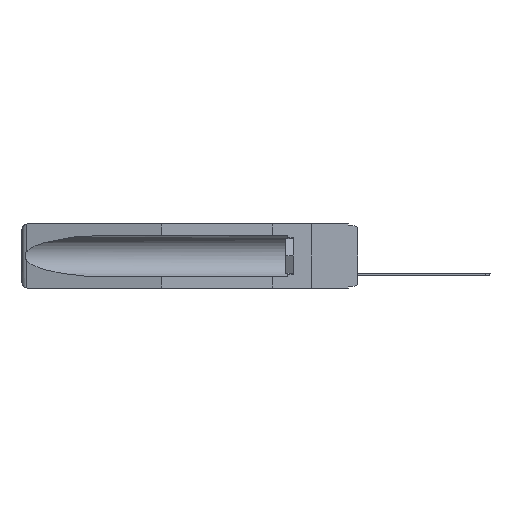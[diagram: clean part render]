
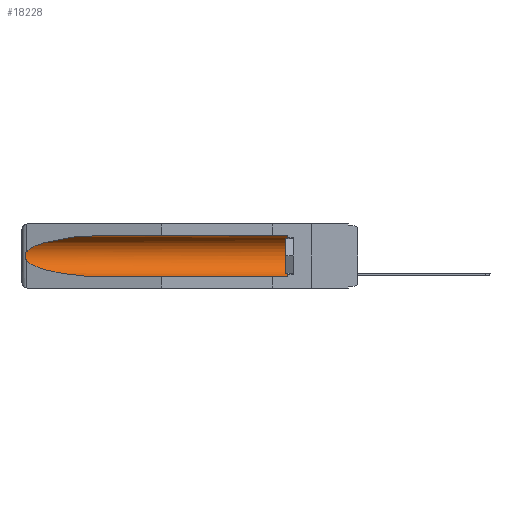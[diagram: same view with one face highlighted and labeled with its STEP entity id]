
A CAD part, left-side view. The second image highlights one B-rep face of the part: STEP entity #18228.
In plain terms, the highlighted cylindrical face has radius 2.857 mm (diameter 5.715 mm), a partial arc.
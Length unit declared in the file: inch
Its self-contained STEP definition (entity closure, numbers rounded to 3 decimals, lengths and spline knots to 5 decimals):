
#122 = CARTESIAN_POINT ( 'NONE',  ( 0.26655, 1.53094, -0.18657 ) ) ;
#272 = ORIENTED_EDGE ( 'NONE', *, *, #1466, .T. ) ;
#1155 =( BOUNDED_CURVE ( )  B_SPLINE_CURVE ( 3, ( #14566, #16086, #17677, #19232 ),
 .UNSPECIFIED., .F., .F. ) 
 B_SPLINE_CURVE_WITH_KNOTS ( ( 4, 4 ),
 ( 0.1948, 1.5708 ),
 .UNSPECIFIED. ) 
 CURVE ( )  GEOMETRIC_REPRESENTATION_ITEM ( )  RATIONAL_B_SPLINE_CURVE ( ( 1., 0.848, 0.848, 1. ) ) 
 REPRESENTATION_ITEM ( '' )  );
#1324 = EDGE_CURVE ( 'NONE', #3491, #7017, #8730, .T. ) ;
#1466 = EDGE_CURVE ( 'NONE', #7017, #9314, #1155, .T. ) ;
#1470 = EDGE_CURVE ( 'NONE', #11580, #15177, #7109, .T. ) ;
#1923 = DIRECTION ( 'NONE',  ( 0., 0., 1. ) ) ;
#1943 = CARTESIAN_POINT ( 'NONE',  ( 0.2673, 1.53269, -0.17917 ) ) ;
#2380 = EDGE_CURVE ( 'NONE', #3036, #3491, #6882, .T. ) ;
#3036 = VERTEX_POINT ( 'NONE', #14897 ) ;
#3089 = EDGE_LOOP ( 'NONE', ( #8557, #5424, #272, #16169, #5481, #16706 ) ) ;
#3181 = AXIS2_PLACEMENT_3D ( 'NONE', #5128, #15964, #6701 ) ;
#3491 = VERTEX_POINT ( 'NONE', #13835 ) ;
#3527 = EDGE_CURVE ( 'NONE', #15177, #3036, #13097, .T. ) ;
#3569 = CARTESIAN_POINT ( 'NONE',  ( 0.155, -0.30754, -0.284 ) ) ;
#4928 = CARTESIAN_POINT ( 'NONE',  ( 0.26537, 1.52718, -0.14972 ) ) ;
#4977 = CARTESIAN_POINT ( 'NONE',  ( 0.155, -0.30754, -0.1715 ) ) ;
#5066 = CARTESIAN_POINT ( 'NONE',  ( 0.26597, 1.5296, -0.19026 ) ) ;
#5128 = CARTESIAN_POINT ( 'NONE',  ( 0.155, 0.126, -0.1715 ) ) ;
#5424 = ORIENTED_EDGE ( 'NONE', *, *, #1324, .T. ) ;
#5481 = ORIENTED_EDGE ( 'NONE', *, *, #1470, .T. ) ;
#5867 = LINE ( 'NONE', #3569, #11201 ) ;
#6054 = VECTOR ( 'NONE', #11794, 39.37008 ) ;
#6504 = CARTESIAN_POINT ( 'NONE',  ( 0.2675, 1.53308, -0.17534 ) ) ;
#6701 = DIRECTION ( 'NONE',  ( 0., 0., 1. ) ) ;
#6882 =( BOUNDED_CURVE ( )  B_SPLINE_CURVE ( 3, ( #18643, #17214, #15638, #9555 ),
 .UNSPECIFIED., .F., .F. ) 
 B_SPLINE_CURVE_WITH_KNOTS ( ( 4, 4 ),
 ( 4.71239, 6.08839 ),
 .UNSPECIFIED. ) 
 CURVE ( )  GEOMETRIC_REPRESENTATION_ITEM ( )  RATIONAL_B_SPLINE_CURVE ( ( 1., 0.848, 0.848, 1. ) ) 
 REPRESENTATION_ITEM ( '' )  );
#7017 = VERTEX_POINT ( 'NONE', #7634 ) ;
#7109 = CIRCLE ( 'NONE', #3181, 0.1125 ) ;
#7634 = CARTESIAN_POINT ( 'NONE',  ( 0.26537, 1.52718, -0.19328 ) ) ;
#8288 = CARTESIAN_POINT ( 'NONE',  ( 0.155, 0.126, -0.059 ) ) ;
#8557 = ORIENTED_EDGE ( 'NONE', *, *, #2380, .T. ) ;
#8730 = B_SPLINE_CURVE_WITH_KNOTS ( 'NONE', 3,
 ( #4928, #9677, #11246, #15752, #12545, #6504, #1943, #122, #5066, #9608 ),
 .UNSPECIFIED., .F., .F.,
 ( 4, 2, 2, 2, 4 ),
 ( 0., 0.00029, 0.00058, 0.00087, 0.00117 ),
 .UNSPECIFIED. ) ;
#9314 = VERTEX_POINT ( 'NONE', #17387 ) ;
#9555 = CARTESIAN_POINT ( 'NONE',  ( 0.26537, 1.52718, -0.14972 ) ) ;
#9608 = CARTESIAN_POINT ( 'NONE',  ( 0.26537, 1.52718, -0.19328 ) ) ;
#9677 = CARTESIAN_POINT ( 'NONE',  ( 0.26597, 1.52961, -0.15275 ) ) ;
#9708 = FACE_OUTER_BOUND ( 'NONE', #3089, .T. ) ;
#9852 = DIRECTION ( 'NONE',  ( 0., 1., 0. ) ) ;
#10766 = AXIS2_PLACEMENT_3D ( 'NONE', #4977, #9852, #1923 ) ;
#10986 = CARTESIAN_POINT ( 'NONE',  ( 0.155, -0.30754, -0.059 ) ) ;
#11201 = VECTOR ( 'NONE', #15965, 39.37008 ) ;
#11246 = CARTESIAN_POINT ( 'NONE',  ( 0.26654, 1.53092, -0.15636 ) ) ;
#11580 = VERTEX_POINT ( 'NONE', #17138 ) ;
#11794 = DIRECTION ( 'NONE',  ( 0., 1., 0. ) ) ;
#12545 = CARTESIAN_POINT ( 'NONE',  ( 0.2675, 1.53308, -0.16763 ) ) ;
#13097 = LINE ( 'NONE', #10986, #6054 ) ;
#13583 = CYLINDRICAL_SURFACE ( 'NONE', #10766, 0.1125 ) ;
#13835 = CARTESIAN_POINT ( 'NONE',  ( 0.26537, 1.52718, -0.14972 ) ) ;
#14566 = CARTESIAN_POINT ( 'NONE',  ( 0.26537, 1.52718, -0.19328 ) ) ;
#14897 = CARTESIAN_POINT ( 'NONE',  ( 0.155, 1.07973, -0.059 ) ) ;
#15177 = VERTEX_POINT ( 'NONE', #8288 ) ;
#15638 = CARTESIAN_POINT ( 'NONE',  ( 0.25451, 1.48313, -0.09465 ) ) ;
#15752 = CARTESIAN_POINT ( 'NONE',  ( 0.2673, 1.5327, -0.16383 ) ) ;
#15964 = DIRECTION ( 'NONE',  ( 0., -1., 0. ) ) ;
#15965 = DIRECTION ( 'NONE',  ( 0., 1., 0. ) ) ;
#16086 = CARTESIAN_POINT ( 'NONE',  ( 0.25451, 1.48313, -0.24835 ) ) ;
#16169 = ORIENTED_EDGE ( 'NONE', *, *, #17586, .F. ) ;
#16706 = ORIENTED_EDGE ( 'NONE', *, *, #3527, .T. ) ;
#17138 = CARTESIAN_POINT ( 'NONE',  ( 0.155, 0.126, -0.284 ) ) ;
#17214 = CARTESIAN_POINT ( 'NONE',  ( 0.21114, 1.30732, -0.059 ) ) ;
#17387 = CARTESIAN_POINT ( 'NONE',  ( 0.155, 1.07973, -0.284 ) ) ;
#17586 = EDGE_CURVE ( 'NONE', #11580, #9314, #5867, .T. ) ;
#17677 = CARTESIAN_POINT ( 'NONE',  ( 0.21114, 1.30732, -0.284 ) ) ;
#18228 = ADVANCED_FACE ( 'NONE', ( #9708 ), #13583, .F. ) ;
#18643 = CARTESIAN_POINT ( 'NONE',  ( 0.155, 1.07973, -0.059 ) ) ;
#19232 = CARTESIAN_POINT ( 'NONE',  ( 0.155, 1.07973, -0.284 ) ) ;
